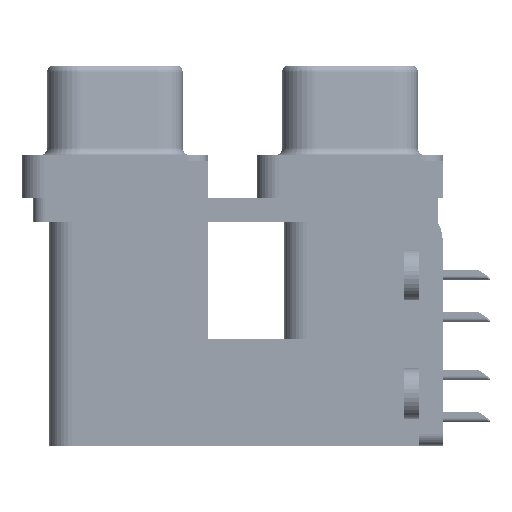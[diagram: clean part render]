
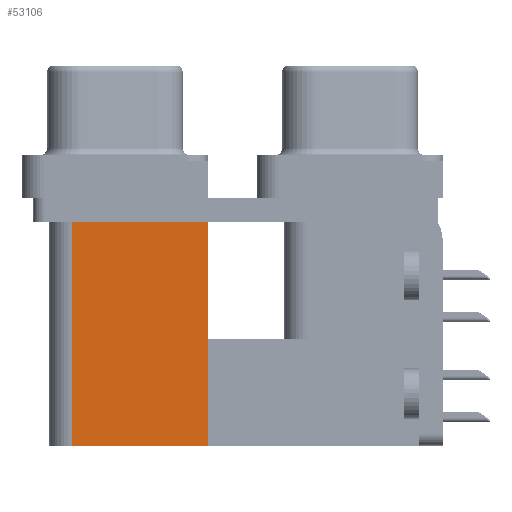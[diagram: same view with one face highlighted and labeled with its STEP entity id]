
A CAD part, left-side view. The second image highlights one B-rep face of the part: STEP entity #53106.
In plain terms, the highlighted planar face has unit normal (-1, 0, 0).
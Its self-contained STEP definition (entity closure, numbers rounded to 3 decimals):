
#254 = DIRECTION ( 'NONE',  ( 0., 0., 1. ) ) ;
#1902 = VECTOR ( 'NONE', #27889, 1000. ) ;
#2811 = LINE ( 'NONE', #12138, #15587 ) ;
#3746 = CARTESIAN_POINT ( 'NONE',  ( 3.79, 9.6, -19.2 ) ) ;
#5120 = VECTOR ( 'NONE', #46736, 1000. ) ;
#7182 = CARTESIAN_POINT ( 'NONE',  ( 3.79, 18.8, -19.2 ) ) ;
#9684 = EDGE_CURVE ( 'NONE', #12233, #23988, #2811, .T. ) ;
#12138 = CARTESIAN_POINT ( 'NONE',  ( 3.79, 18.8, -19.2 ) ) ;
#12233 = VERTEX_POINT ( 'NONE', #7182 ) ;
#14395 = EDGE_CURVE ( 'NONE', #38074, #12233, #47007, .T. ) ;
#15419 = CARTESIAN_POINT ( 'NONE',  ( 3.79, 9.6, -19.2 ) ) ;
#15587 = VECTOR ( 'NONE', #254, 1000. ) ;
#16485 = EDGE_CURVE ( 'NONE', #26241, #23988, #41578, .T. ) ;
#17863 = CARTESIAN_POINT ( 'NONE',  ( 3.79, 18.8, -2.5 ) ) ;
#23988 = VERTEX_POINT ( 'NONE', #17863 ) ;
#25042 = CARTESIAN_POINT ( 'NONE',  ( 3.79, 9.6, -2.5 ) ) ;
#26241 = VERTEX_POINT ( 'NONE', #25042 ) ;
#26568 = DIRECTION ( 'NONE',  ( 1., 0., 0. ) ) ;
#27889 = DIRECTION ( 'NONE',  ( 0., 0., 1. ) ) ;
#27896 = EDGE_LOOP ( 'NONE', ( #45566, #40684, #30376, #41627 ) ) ;
#30376 = ORIENTED_EDGE ( 'NONE', *, *, #14395, .F. ) ;
#31926 = LINE ( 'NONE', #48380, #1902 ) ;
#37258 = DIRECTION ( 'NONE',  ( 0., 1., 0. ) ) ;
#38074 = VERTEX_POINT ( 'NONE', #3746 ) ;
#39167 = CARTESIAN_POINT ( 'NONE',  ( 3.79, 9.6, -19.2 ) ) ;
#39973 = PLANE ( 'NONE',  #42744 ) ;
#40684 = ORIENTED_EDGE ( 'NONE', *, *, #9684, .F. ) ;
#41578 = LINE ( 'NONE', #49410, #43889 ) ;
#41627 = ORIENTED_EDGE ( 'NONE', *, *, #44792, .T. ) ;
#42744 = AXIS2_PLACEMENT_3D ( 'NONE', #15419, #26568, #52640 ) ;
#43889 = VECTOR ( 'NONE', #37258, 1000. ) ;
#44792 = EDGE_CURVE ( 'NONE', #38074, #26241, #31926, .T. ) ;
#45566 = ORIENTED_EDGE ( 'NONE', *, *, #16485, .T. ) ;
#46736 = DIRECTION ( 'NONE',  ( 0., 1., 0. ) ) ;
#47007 = LINE ( 'NONE', #39167, #5120 ) ;
#48380 = CARTESIAN_POINT ( 'NONE',  ( 3.79, 9.6, -19.2 ) ) ;
#49410 = CARTESIAN_POINT ( 'NONE',  ( 3.79, 9.6, -2.5 ) ) ;
#52381 = FACE_OUTER_BOUND ( 'NONE', #27896, .T. ) ;
#52640 = DIRECTION ( 'NONE',  ( 0., 0., -1. ) ) ;
#53106 = ADVANCED_FACE ( 'NONE', ( #52381 ), #39973, .F. ) ;
